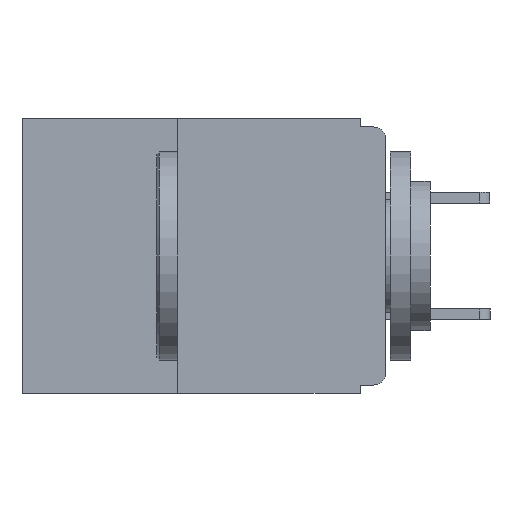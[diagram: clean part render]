
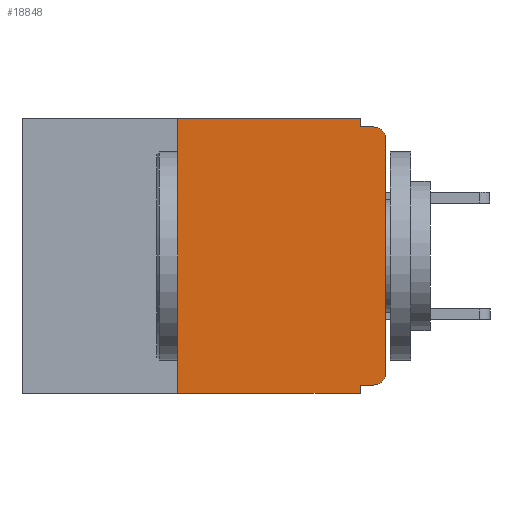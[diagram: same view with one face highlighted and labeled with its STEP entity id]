
A CAD part, left-side view. The second image highlights one B-rep face of the part: STEP entity #18848.
In plain terms, the highlighted planar face has unit normal (-1, 0, 0).
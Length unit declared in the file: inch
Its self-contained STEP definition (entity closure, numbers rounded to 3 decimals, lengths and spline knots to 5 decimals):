
#223 = DIRECTION ( 'NONE',  ( 0., -1., 0. ) ) ;
#338 = DIRECTION ( 'NONE',  ( 0., 0., 1. ) ) ;
#544 = CIRCLE ( 'NONE', #5809, 0.015 ) ;
#791 = CARTESIAN_POINT ( 'NONE',  ( 0., 0.25, -0.33 ) ) ;
#817 = VERTEX_POINT ( 'NONE', #19724 ) ;
#1051 = LINE ( 'NONE', #8532, #9747 ) ;
#1053 = EDGE_CURVE ( 'NONE', #20467, #4376, #8313, .T. ) ;
#1088 = CARTESIAN_POINT ( 'NONE',  ( 0., 0., -0.32 ) ) ;
#1917 = ORIENTED_EDGE ( 'NONE', *, *, #11330, .F. ) ;
#2340 = CARTESIAN_POINT ( 'NONE',  ( 0., 0.015, -0.025 ) ) ;
#2774 = AXIS2_PLACEMENT_3D ( 'NONE', #2340, #14251, #4074 ) ;
#2927 = LINE ( 'NONE', #13331, #20230 ) ;
#3481 = CARTESIAN_POINT ( 'NONE',  ( 0., 0.031, 0. ) ) ;
#4074 = DIRECTION ( 'NONE',  ( 0., 0., -1. ) ) ;
#4376 = VERTEX_POINT ( 'NONE', #5310 ) ;
#4381 = VECTOR ( 'NONE', #14754, 39.37008 ) ;
#4745 = EDGE_CURVE ( 'NONE', #9428, #817, #15030, .T. ) ;
#4774 = CARTESIAN_POINT ( 'NONE',  ( 0., 0.25, -0.33 ) ) ;
#5041 = DIRECTION ( 'NONE',  ( 0., 0., -1. ) ) ;
#5199 = DIRECTION ( 'NONE',  ( 0., 0., -1. ) ) ;
#5205 = DIRECTION ( 'NONE',  ( -1., 0., 0. ) ) ;
#5254 = CARTESIAN_POINT ( 'NONE',  ( 0., 0.015, -0.305 ) ) ;
#5310 = CARTESIAN_POINT ( 'NONE',  ( 0., 0., -0.025 ) ) ;
#5561 = CARTESIAN_POINT ( 'NONE',  ( 0., 0.031, -0.33 ) ) ;
#5742 = VECTOR ( 'NONE', #223, 39.37008 ) ;
#5809 = AXIS2_PLACEMENT_3D ( 'NONE', #5254, #5205, #5199 ) ;
#5955 = EDGE_CURVE ( 'NONE', #17062, #20467, #544, .T. ) ;
#6073 = CARTESIAN_POINT ( 'NONE',  ( 0., 0.437, -0.33 ) ) ;
#6249 = CARTESIAN_POINT ( 'NONE',  ( 0., 0.015, -0.32 ) ) ;
#6553 = DIRECTION ( 'NONE',  ( 0., -1., 0. ) ) ;
#6903 = ORIENTED_EDGE ( 'NONE', *, *, #17616, .T. ) ;
#7044 = CARTESIAN_POINT ( 'NONE',  ( 0., 0.031, 0. ) ) ;
#7770 = VECTOR ( 'NONE', #8025, 39.37008 ) ;
#7844 = DIRECTION ( 'NONE',  ( 0., -1., 0. ) ) ;
#7922 = FACE_OUTER_BOUND ( 'NONE', #21248, .T. ) ;
#8025 = DIRECTION ( 'NONE',  ( 0., 0., 1. ) ) ;
#8042 = CARTESIAN_POINT ( 'NONE',  ( 0., 0.031, -0.32 ) ) ;
#8313 = LINE ( 'NONE', #9048, #7770 ) ;
#8483 = CARTESIAN_POINT ( 'NONE',  ( 0., 0.437, 0. ) ) ;
#8532 = CARTESIAN_POINT ( 'NONE',  ( 0., 0.031, -0.33 ) ) ;
#8824 = DIRECTION ( 'NONE',  ( 0., 0., -1. ) ) ;
#8934 = ORIENTED_EDGE ( 'NONE', *, *, #14647, .T. ) ;
#9048 = CARTESIAN_POINT ( 'NONE',  ( 0., 0., 0. ) ) ;
#9428 = VERTEX_POINT ( 'NONE', #4774 ) ;
#9747 = VECTOR ( 'NONE', #5041, 39.37008 ) ;
#9867 = CARTESIAN_POINT ( 'NONE',  ( 0., 0., -0.305 ) ) ;
#10150 = VERTEX_POINT ( 'NONE', #5561 ) ;
#10199 = DIRECTION ( 'NONE',  ( 1., 0., 0. ) ) ;
#10784 = ORIENTED_EDGE ( 'NONE', *, *, #18497, .F. ) ;
#11102 = VECTOR ( 'NONE', #8824, 39.37008 ) ;
#11330 = EDGE_CURVE ( 'NONE', #18772, #14549, #2927, .T. ) ;
#11453 = VERTEX_POINT ( 'NONE', #3481 ) ;
#11626 = LINE ( 'NONE', #7044, #11102 ) ;
#11999 = VECTOR ( 'NONE', #7844, 39.37008 ) ;
#12527 = LINE ( 'NONE', #6073, #11999 ) ;
#13130 = VERTEX_POINT ( 'NONE', #8042 ) ;
#13331 = CARTESIAN_POINT ( 'NONE',  ( 0., 0., -0.01 ) ) ;
#14251 = DIRECTION ( 'NONE',  ( -1., 0., 0. ) ) ;
#14549 = VERTEX_POINT ( 'NONE', #20450 ) ;
#14647 = EDGE_CURVE ( 'NONE', #4376, #14549, #18837, .T. ) ;
#14754 = DIRECTION ( 'NONE',  ( 0., 1., 0. ) ) ;
#15030 = LINE ( 'NONE', #791, #18863 ) ;
#15037 = ORIENTED_EDGE ( 'NONE', *, *, #1053, .T. ) ;
#15296 = LINE ( 'NONE', #18745, #5742 ) ;
#16113 = EDGE_CURVE ( 'NONE', #11453, #18772, #11626, .T. ) ;
#17062 = VERTEX_POINT ( 'NONE', #6249 ) ;
#17235 = ORIENTED_EDGE ( 'NONE', *, *, #19783, .F. ) ;
#17616 = EDGE_CURVE ( 'NONE', #9428, #10150, #12527, .T. ) ;
#17853 = LINE ( 'NONE', #1088, #4381 ) ;
#18298 = ORIENTED_EDGE ( 'NONE', *, *, #5955, .T. ) ;
#18453 = PLANE ( 'NONE',  #20522 ) ;
#18497 = EDGE_CURVE ( 'NONE', #817, #11453, #15296, .T. ) ;
#18730 = ORIENTED_EDGE ( 'NONE', *, *, #21221, .F. ) ;
#18745 = CARTESIAN_POINT ( 'NONE',  ( 0., 0.437, 0. ) ) ;
#18772 = VERTEX_POINT ( 'NONE', #21093 ) ;
#18837 = CIRCLE ( 'NONE', #2774, 0.015 ) ;
#18848 = ADVANCED_FACE ( 'NONE', ( #7922 ), #18453, .F. ) ;
#18863 = VECTOR ( 'NONE', #338, 39.37008 ) ;
#18946 = ORIENTED_EDGE ( 'NONE', *, *, #4745, .F. ) ;
#19488 = ORIENTED_EDGE ( 'NONE', *, *, #16113, .F. ) ;
#19724 = CARTESIAN_POINT ( 'NONE',  ( 0., 0.25, 0. ) ) ;
#19783 = EDGE_CURVE ( 'NONE', #17062, #13130, #17853, .T. ) ;
#20230 = VECTOR ( 'NONE', #6553, 39.37008 ) ;
#20450 = CARTESIAN_POINT ( 'NONE',  ( 0., 0.015, -0.01 ) ) ;
#20467 = VERTEX_POINT ( 'NONE', #9867 ) ;
#20522 = AXIS2_PLACEMENT_3D ( 'NONE', #8483, #10199, #21634 ) ;
#21093 = CARTESIAN_POINT ( 'NONE',  ( 0., 0.031, -0.01 ) ) ;
#21221 = EDGE_CURVE ( 'NONE', #13130, #10150, #1051, .T. ) ;
#21248 = EDGE_LOOP ( 'NONE', ( #15037, #8934, #1917, #19488, #10784, #18946, #6903, #18730, #17235, #18298 ) ) ;
#21634 = DIRECTION ( 'NONE',  ( 0., 0., -1. ) ) ;
